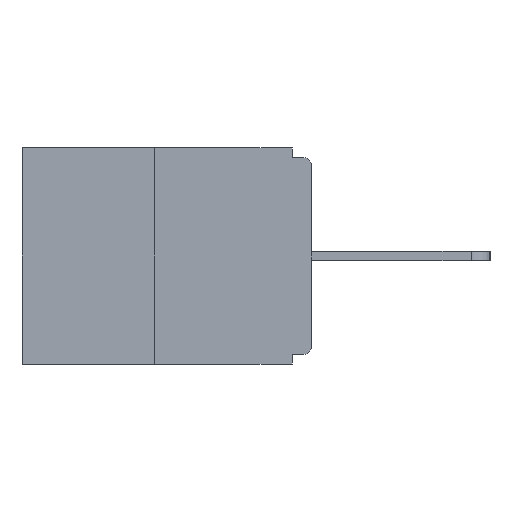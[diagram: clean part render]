
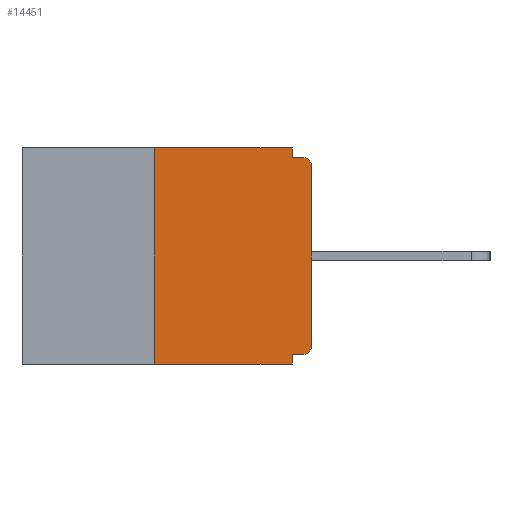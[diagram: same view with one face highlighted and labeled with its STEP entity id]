
A CAD part, left-side view. The second image highlights one B-rep face of the part: STEP entity #14451.
In plain terms, the highlighted planar face has unit normal (-1, 0, 0).
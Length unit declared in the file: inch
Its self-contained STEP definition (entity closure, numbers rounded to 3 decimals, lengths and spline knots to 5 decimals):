
#1183 = EDGE_LOOP ( 'NONE', ( #6622, #6634, #7081, #7128, #7325, #7600, #8260, #8866, #9083, #9308 ) ) ;
#1210 = CARTESIAN_POINT ( 'NONE',  ( 0., 0.015, -0.328 ) ) ;
#1264 = DIRECTION ( 'NONE',  ( 0., 0., -1. ) ) ;
#1687 = CARTESIAN_POINT ( 'NONE',  ( 0., 0.25, 0. ) ) ;
#1734 = AXIS2_PLACEMENT_3D ( 'NONE', #3009, #14881, #7111 ) ;
#2935 = EDGE_CURVE ( 'NONE', #16925, #5838, #10837, .T. ) ;
#3009 = CARTESIAN_POINT ( 'NONE',  ( 0., 0.46, 0. ) ) ;
#3134 = DIRECTION ( 'NONE',  ( 0., 0., 1. ) ) ;
#3223 = VECTOR ( 'NONE', #14060, 39.37008 ) ;
#3457 = FACE_OUTER_BOUND ( 'NONE', #1183, .T. ) ;
#3563 = EDGE_CURVE ( 'NONE', #13297, #6006, #12203, .T. ) ;
#3624 = CARTESIAN_POINT ( 'NONE',  ( 0., 0., -0.328 ) ) ;
#3764 = DIRECTION ( 'NONE',  ( -1., 0., 0. ) ) ;
#3803 = VECTOR ( 'NONE', #8160, 39.37008 ) ;
#3892 = DIRECTION ( 'NONE',  ( 0., 0., 1. ) ) ;
#3971 = CARTESIAN_POINT ( 'NONE',  ( 0., 0.46, -0.343 ) ) ;
#4289 = DIRECTION ( 'NONE',  ( -1., 0., 0. ) ) ;
#4551 = CARTESIAN_POINT ( 'NONE',  ( 0., 0., -0.03 ) ) ;
#4572 = EDGE_CURVE ( 'NONE', #12713, #12716, #16632, .T. ) ;
#4966 = CARTESIAN_POINT ( 'NONE',  ( 0., 0.031, -0.343 ) ) ;
#5077 = AXIS2_PLACEMENT_3D ( 'NONE', #11637, #3764, #12926 ) ;
#5081 = CARTESIAN_POINT ( 'NONE',  ( 0., 0., 0. ) ) ;
#5347 = VECTOR ( 'NONE', #8507, 39.37008 ) ;
#5508 = EDGE_CURVE ( 'NONE', #15130, #15728, #6071, .T. ) ;
#5745 = PLANE ( 'NONE',  #1734 ) ;
#5838 = VERTEX_POINT ( 'NONE', #4966 ) ;
#6006 = VERTEX_POINT ( 'NONE', #13800 ) ;
#6058 = VERTEX_POINT ( 'NONE', #7351 ) ;
#6071 = LINE ( 'NONE', #5081, #9965 ) ;
#6298 = VECTOR ( 'NONE', #13476, 39.37008 ) ;
#6430 = CARTESIAN_POINT ( 'NONE',  ( 0., 0.25, 0. ) ) ;
#6622 = ORIENTED_EDGE ( 'NONE', *, *, #14689, .F. ) ;
#6634 = ORIENTED_EDGE ( 'NONE', *, *, #8868, .F. ) ;
#7081 = ORIENTED_EDGE ( 'NONE', *, *, #2935, .T. ) ;
#7111 = DIRECTION ( 'NONE',  ( 0., 0., -1. ) ) ;
#7128 = ORIENTED_EDGE ( 'NONE', *, *, #11581, .F. ) ;
#7134 = CIRCLE ( 'NONE', #14749, 0.015 ) ;
#7325 = ORIENTED_EDGE ( 'NONE', *, *, #3563, .F. ) ;
#7351 = CARTESIAN_POINT ( 'NONE',  ( 0., 0.015, -0.015 ) ) ;
#7600 = ORIENTED_EDGE ( 'NONE', *, *, #12763, .T. ) ;
#7777 = VERTEX_POINT ( 'NONE', #6430 ) ;
#8000 = VECTOR ( 'NONE', #3134, 39.37008 ) ;
#8160 = DIRECTION ( 'NONE',  ( 0., -1., 0. ) ) ;
#8260 = ORIENTED_EDGE ( 'NONE', *, *, #5508, .T. ) ;
#8507 = DIRECTION ( 'NONE',  ( 0., -1., 0. ) ) ;
#8592 = LINE ( 'NONE', #17140, #15090 ) ;
#8866 = ORIENTED_EDGE ( 'NONE', *, *, #10299, .T. ) ;
#8868 = EDGE_CURVE ( 'NONE', #16925, #7777, #14908, .T. ) ;
#9083 = ORIENTED_EDGE ( 'NONE', *, *, #15089, .F. ) ;
#9243 = CIRCLE ( 'NONE', #5077, 0.015 ) ;
#9308 = ORIENTED_EDGE ( 'NONE', *, *, #4572, .F. ) ;
#9965 = VECTOR ( 'NONE', #3892, 39.37008 ) ;
#9988 = CARTESIAN_POINT ( 'NONE',  ( 0., 0.25, -0.343 ) ) ;
#10299 = EDGE_CURVE ( 'NONE', #15728, #6058, #9243, .T. ) ;
#10741 = CARTESIAN_POINT ( 'NONE',  ( 0., 0.031, -0.015 ) ) ;
#10837 = LINE ( 'NONE', #3971, #3803 ) ;
#11581 = EDGE_CURVE ( 'NONE', #6006, #5838, #8592, .T. ) ;
#11637 = CARTESIAN_POINT ( 'NONE',  ( 0., 0.015, -0.03 ) ) ;
#12118 = CARTESIAN_POINT ( 'NONE',  ( 0., 0.015, -0.313 ) ) ;
#12203 = LINE ( 'NONE', #3624, #15276 ) ;
#12713 = VERTEX_POINT ( 'NONE', #15886 ) ;
#12716 = VERTEX_POINT ( 'NONE', #10741 ) ;
#12737 = CARTESIAN_POINT ( 'NONE',  ( 0., 0.46, 0. ) ) ;
#12763 = EDGE_CURVE ( 'NONE', #13297, #15130, #7134, .T. ) ;
#12926 = DIRECTION ( 'NONE',  ( 0., 0., -1. ) ) ;
#13214 = DIRECTION ( 'NONE',  ( 0., 1., 0. ) ) ;
#13297 = VERTEX_POINT ( 'NONE', #1210 ) ;
#13422 = DIRECTION ( 'NONE',  ( 0., 0., -1. ) ) ;
#13476 = DIRECTION ( 'NONE',  ( 0., 0., -1. ) ) ;
#13653 = CARTESIAN_POINT ( 'NONE',  ( 0., 0.031, 0. ) ) ;
#13800 = CARTESIAN_POINT ( 'NONE',  ( 0., 0.031, -0.328 ) ) ;
#14060 = DIRECTION ( 'NONE',  ( 0., -1., 0. ) ) ;
#14451 = ADVANCED_FACE ( 'NONE', ( #3457 ), #5745, .F. ) ;
#14689 = EDGE_CURVE ( 'NONE', #7777, #12713, #17170, .T. ) ;
#14749 = AXIS2_PLACEMENT_3D ( 'NONE', #12118, #4289, #13422 ) ;
#14881 = DIRECTION ( 'NONE',  ( 1., 0., 0. ) ) ;
#14908 = LINE ( 'NONE', #1687, #8000 ) ;
#14969 = CARTESIAN_POINT ( 'NONE',  ( 0., 0., -0.015 ) ) ;
#15025 = CARTESIAN_POINT ( 'NONE',  ( 0., 0., -0.313 ) ) ;
#15089 = EDGE_CURVE ( 'NONE', #12716, #6058, #16170, .T. ) ;
#15090 = VECTOR ( 'NONE', #1264, 39.37008 ) ;
#15130 = VERTEX_POINT ( 'NONE', #15025 ) ;
#15276 = VECTOR ( 'NONE', #13214, 39.37008 ) ;
#15728 = VERTEX_POINT ( 'NONE', #4551 ) ;
#15886 = CARTESIAN_POINT ( 'NONE',  ( 0., 0.031, 0. ) ) ;
#16170 = LINE ( 'NONE', #14969, #5347 ) ;
#16632 = LINE ( 'NONE', #13653, #6298 ) ;
#16925 = VERTEX_POINT ( 'NONE', #9988 ) ;
#17140 = CARTESIAN_POINT ( 'NONE',  ( 0., 0.031, -0.343 ) ) ;
#17170 = LINE ( 'NONE', #12737, #3223 ) ;
